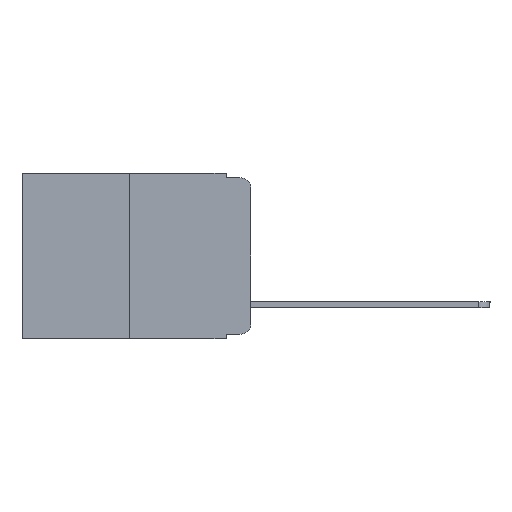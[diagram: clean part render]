
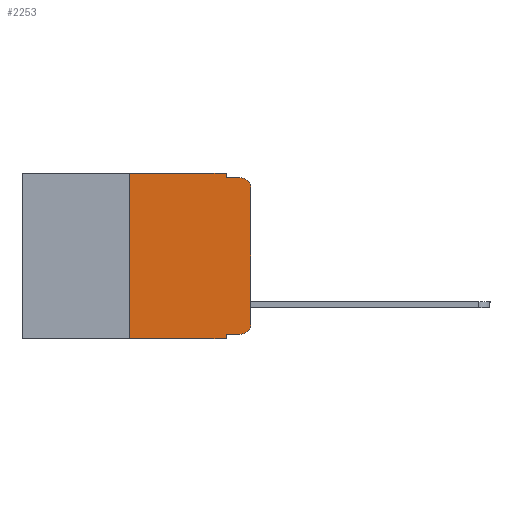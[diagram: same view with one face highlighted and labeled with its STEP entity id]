
A CAD part, left-side view. The second image highlights one B-rep face of the part: STEP entity #2253.
In plain terms, the highlighted planar face has unit normal (-1, 0, 0).
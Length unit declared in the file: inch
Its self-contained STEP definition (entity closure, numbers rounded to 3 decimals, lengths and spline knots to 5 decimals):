
#891 = DIRECTION ( 'NONE',  ( 0., -1., 0. ) ) ;
#996 = EDGE_CURVE ( 'NONE', #20285, #4646, #16385, .T. ) ;
#2253 = ADVANCED_FACE ( 'NONE', ( #16534 ), #23187, .F. ) ;
#2919 = VECTOR ( 'NONE', #17325, 39.37008 ) ;
#2960 = VECTOR ( 'NONE', #891, 39.37008 ) ;
#3498 = CIRCLE ( 'NONE', #25641, 0.02 ) ;
#4386 = CARTESIAN_POINT ( 'NONE',  ( 0., 0.02, -0.333 ) ) ;
#4544 = CARTESIAN_POINT ( 'NONE',  ( 0., 0.473, 0. ) ) ;
#4646 = VERTEX_POINT ( 'NONE', #4386 ) ;
#5074 = CARTESIAN_POINT ( 'NONE',  ( 0., 0.25, -0.343 ) ) ;
#5570 = CARTESIAN_POINT ( 'NONE',  ( 0., 0.051, 0. ) ) ;
#5578 = CARTESIAN_POINT ( 'NONE',  ( 0., 0., 0. ) ) ;
#5643 = ORIENTED_EDGE ( 'NONE', *, *, #16635, .T. ) ;
#5791 = VECTOR ( 'NONE', #24090, 39.37008 ) ;
#5812 = CARTESIAN_POINT ( 'NONE',  ( 0., 0., -0.313 ) ) ;
#5967 = VERTEX_POINT ( 'NONE', #19107 ) ;
#6109 = VERTEX_POINT ( 'NONE', #5074 ) ;
#6239 = CARTESIAN_POINT ( 'NONE',  ( 0., 0.02, -0.01 ) ) ;
#6270 = DIRECTION ( 'NONE',  ( 0., -1., 0. ) ) ;
#6360 = CARTESIAN_POINT ( 'NONE',  ( 0., 0.051, -0.01 ) ) ;
#6540 = CARTESIAN_POINT ( 'NONE',  ( 0., 0.473, 0. ) ) ;
#6621 = CARTESIAN_POINT ( 'NONE',  ( 0., 0.25, 0. ) ) ;
#6631 = DIRECTION ( 'NONE',  ( 0., 0., -1. ) ) ;
#6800 = EDGE_CURVE ( 'NONE', #14741, #22719, #19559, .T. ) ;
#7498 = VERTEX_POINT ( 'NONE', #5570 ) ;
#7833 = ORIENTED_EDGE ( 'NONE', *, *, #6800, .F. ) ;
#8839 = CARTESIAN_POINT ( 'NONE',  ( 0., 0.02, -0.03 ) ) ;
#8932 = LINE ( 'NONE', #10427, #19041 ) ;
#9483 = AXIS2_PLACEMENT_3D ( 'NONE', #22270, #24445, #14515 ) ;
#9875 = VERTEX_POINT ( 'NONE', #5812 ) ;
#10427 = CARTESIAN_POINT ( 'NONE',  ( 0., 0.051, 0. ) ) ;
#10863 = DIRECTION ( 'NONE',  ( -1., 0., 0. ) ) ;
#11244 = CIRCLE ( 'NONE', #9483, 0.02 ) ;
#11251 = CARTESIAN_POINT ( 'NONE',  ( 0., 0.051, -0.01 ) ) ;
#11332 = CARTESIAN_POINT ( 'NONE',  ( 0., 0.051, -0.333 ) ) ;
#11706 = EDGE_CURVE ( 'NONE', #6109, #17211, #25256, .T. ) ;
#11947 = VECTOR ( 'NONE', #22677, 39.37008 ) ;
#12394 = ORIENTED_EDGE ( 'NONE', *, *, #20837, .T. ) ;
#12965 = LINE ( 'NONE', #19234, #2919 ) ;
#13049 = DIRECTION ( 'NONE',  ( 0., 0., -1. ) ) ;
#13190 = LINE ( 'NONE', #17548, #15983 ) ;
#13200 = ORIENTED_EDGE ( 'NONE', *, *, #23710, .F. ) ;
#13492 = ORIENTED_EDGE ( 'NONE', *, *, #996, .T. ) ;
#13564 = ORIENTED_EDGE ( 'NONE', *, *, #11706, .F. ) ;
#13571 = EDGE_CURVE ( 'NONE', #6109, #5967, #12965, .T. ) ;
#14056 = VERTEX_POINT ( 'NONE', #17970 ) ;
#14352 = DIRECTION ( 'NONE',  ( 0., -1., 0. ) ) ;
#14515 = DIRECTION ( 'NONE',  ( 0., 0., -1. ) ) ;
#14529 = VECTOR ( 'NONE', #14352, 39.37008 ) ;
#14741 = VERTEX_POINT ( 'NONE', #6360 ) ;
#15983 = VECTOR ( 'NONE', #21505, 39.37008 ) ;
#16385 = LINE ( 'NONE', #16666, #14529 ) ;
#16534 = FACE_OUTER_BOUND ( 'NONE', #20731, .T. ) ;
#16540 = ORIENTED_EDGE ( 'NONE', *, *, #25696, .T. ) ;
#16635 = EDGE_CURVE ( 'NONE', #4646, #9875, #11244, .T. ) ;
#16666 = CARTESIAN_POINT ( 'NONE',  ( 0., 0.051, -0.333 ) ) ;
#17183 = CARTESIAN_POINT ( 'NONE',  ( 0., 0.25, 0. ) ) ;
#17211 = VERTEX_POINT ( 'NONE', #17183 ) ;
#17325 = DIRECTION ( 'NONE',  ( 0., -1., 0. ) ) ;
#17548 = CARTESIAN_POINT ( 'NONE',  ( 0., 0.051, 0. ) ) ;
#17970 = CARTESIAN_POINT ( 'NONE',  ( 0., 0., -0.03 ) ) ;
#18516 = ORIENTED_EDGE ( 'NONE', *, *, #23748, .F. ) ;
#18919 = AXIS2_PLACEMENT_3D ( 'NONE', #4544, #24958, #21144 ) ;
#19041 = VECTOR ( 'NONE', #6631, 39.37008 ) ;
#19107 = CARTESIAN_POINT ( 'NONE',  ( 0., 0.051, -0.343 ) ) ;
#19234 = CARTESIAN_POINT ( 'NONE',  ( 0., 0.473, -0.343 ) ) ;
#19559 = LINE ( 'NONE', #11251, #2960 ) ;
#20285 = VERTEX_POINT ( 'NONE', #11332 ) ;
#20612 = ORIENTED_EDGE ( 'NONE', *, *, #23500, .F. ) ;
#20731 = EDGE_LOOP ( 'NONE', ( #12394, #16540, #7833, #13200, #20612, #13564, #26043, #18516, #13492, #5643 ) ) ;
#20837 = EDGE_CURVE ( 'NONE', #9875, #14056, #21915, .T. ) ;
#21144 = DIRECTION ( 'NONE',  ( 0., 0., -1. ) ) ;
#21505 = DIRECTION ( 'NONE',  ( 0., 0., -1. ) ) ;
#21915 = LINE ( 'NONE', #5578, #5791 ) ;
#22270 = CARTESIAN_POINT ( 'NONE',  ( 0., 0.02, -0.313 ) ) ;
#22677 = DIRECTION ( 'NONE',  ( 0., 0., 1. ) ) ;
#22719 = VERTEX_POINT ( 'NONE', #6239 ) ;
#23187 = PLANE ( 'NONE',  #18919 ) ;
#23500 = EDGE_CURVE ( 'NONE', #17211, #7498, #24510, .T. ) ;
#23710 = EDGE_CURVE ( 'NONE', #7498, #14741, #13190, .T. ) ;
#23748 = EDGE_CURVE ( 'NONE', #20285, #5967, #8932, .T. ) ;
#24090 = DIRECTION ( 'NONE',  ( 0., 0., 1. ) ) ;
#24445 = DIRECTION ( 'NONE',  ( -1., 0., 0. ) ) ;
#24510 = LINE ( 'NONE', #6540, #26368 ) ;
#24958 = DIRECTION ( 'NONE',  ( 1., 0., 0. ) ) ;
#25256 = LINE ( 'NONE', #6621, #11947 ) ;
#25641 = AXIS2_PLACEMENT_3D ( 'NONE', #8839, #10863, #13049 ) ;
#25696 = EDGE_CURVE ( 'NONE', #14056, #22719, #3498, .T. ) ;
#26043 = ORIENTED_EDGE ( 'NONE', *, *, #13571, .T. ) ;
#26368 = VECTOR ( 'NONE', #6270, 39.37008 ) ;
